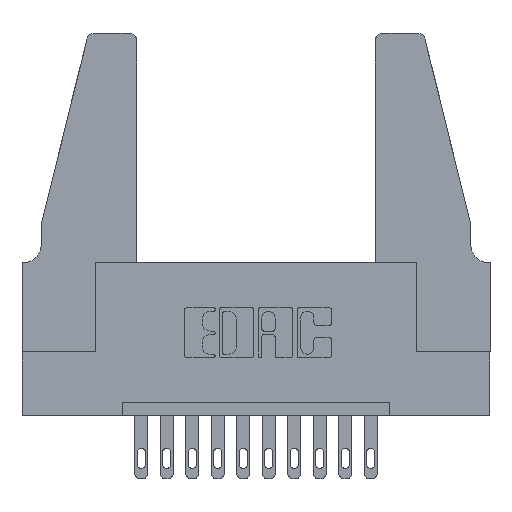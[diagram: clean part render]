
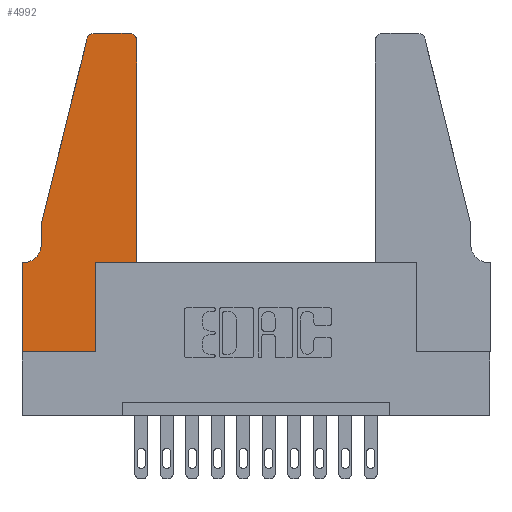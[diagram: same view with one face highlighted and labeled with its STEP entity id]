
A CAD part, top view. The second image highlights one B-rep face of the part: STEP entity #4992.
In plain terms, the highlighted planar face has unit normal (0, 0, 1).
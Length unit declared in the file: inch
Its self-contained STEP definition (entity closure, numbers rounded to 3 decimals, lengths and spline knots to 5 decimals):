
#317 = EDGE_LOOP ( 'NONE', ( #1395, #3519, #5542, #6580, #8007, #12142, #10246, #6247, #4694, #13331, #13480, #3864 ) ) ;
#408 = CARTESIAN_POINT ( 'NONE',  ( 0., 0.35, 0.37 ) ) ;
#472 = LINE ( 'NONE', #2294, #2865 ) ;
#598 = EDGE_CURVE ( 'NONE', #11204, #2477, #13326, .T. ) ;
#665 = EDGE_CURVE ( 'NONE', #9287, #4474, #9991, .T. ) ;
#851 = VECTOR ( 'NONE', #13120, 39.37008 ) ;
#853 = VECTOR ( 'NONE', #7889, 39.37008 ) ;
#1006 = DIRECTION ( 'NONE',  ( -1., 0., 0. ) ) ;
#1030 = EDGE_CURVE ( 'NONE', #8164, #5108, #3789, .T. ) ;
#1097 = CARTESIAN_POINT ( 'NONE',  ( 0.2865, 0.35, 0.37 ) ) ;
#1222 = DIRECTION ( 'NONE',  ( 0., -1., 0. ) ) ;
#1226 = CARTESIAN_POINT ( 'NONE',  ( 0.25487, 1.22718, 0.37 ) ) ;
#1299 = CARTESIAN_POINT ( 'NONE',  ( 0.2605, 1.25, 0.37 ) ) ;
#1341 = CARTESIAN_POINT ( 'NONE',  ( 0.4205, 1.25, 0.37 ) ) ;
#1350 = DIRECTION ( 'NONE',  ( -1., 0., 0. ) ) ;
#1395 = ORIENTED_EDGE ( 'NONE', *, *, #1030, .T. ) ;
#1407 = VERTEX_POINT ( 'NONE', #7362 ) ;
#1557 = CARTESIAN_POINT ( 'NONE',  ( 0., 0., 0.37 ) ) ;
#1615 = VERTEX_POINT ( 'NONE', #1226 ) ;
#1928 = VECTOR ( 'NONE', #12674, 39.37008 ) ;
#2141 = VERTEX_POINT ( 'NONE', #2352 ) ;
#2143 = CIRCLE ( 'NONE', #5082, 0.07 ) ;
#2294 = CARTESIAN_POINT ( 'NONE',  ( 0.0755, 0.5, 0.37 ) ) ;
#2352 = CARTESIAN_POINT ( 'NONE',  ( 0.0755, 0.5, 0.37 ) ) ;
#2477 = VERTEX_POINT ( 'NONE', #12676 ) ;
#2831 = DIRECTION ( 'NONE',  ( 1., 0., 0. ) ) ;
#2865 = VECTOR ( 'NONE', #1222, 39.37008 ) ;
#2970 = EDGE_CURVE ( 'NONE', #2477, #6787, #6252, .T. ) ;
#3180 = DIRECTION ( 'NONE',  ( 0., 0., 1. ) ) ;
#3229 = LINE ( 'NONE', #3492, #853 ) ;
#3268 = EDGE_CURVE ( 'NONE', #1615, #2141, #9813, .T. ) ;
#3292 = CARTESIAN_POINT ( 'NONE',  ( 0.0055, 0.42, 0.37 ) ) ;
#3492 = CARTESIAN_POINT ( 'NONE',  ( 0.4505, 0.35, 0.37 ) ) ;
#3519 = ORIENTED_EDGE ( 'NONE', *, *, #11534, .T. ) ;
#3631 = DIRECTION ( 'NONE',  ( -1., 0., 0. ) ) ;
#3654 = CARTESIAN_POINT ( 'NONE',  ( 0.4205, 1.22, 0.37 ) ) ;
#3789 = LINE ( 'NONE', #1299, #10139 ) ;
#3864 = ORIENTED_EDGE ( 'NONE', *, *, #13482, .T. ) ;
#3940 = LINE ( 'NONE', #5899, #7748 ) ;
#4137 = CARTESIAN_POINT ( 'NONE',  ( 0.0755, 0.5, 0.37 ) ) ;
#4387 = LINE ( 'NONE', #5667, #851 ) ;
#4416 = AXIS2_PLACEMENT_3D ( 'NONE', #13849, #3180, #9418 ) ;
#4474 = VERTEX_POINT ( 'NONE', #7382 ) ;
#4694 = ORIENTED_EDGE ( 'NONE', *, *, #665, .T. ) ;
#4734 = DIRECTION ( 'NONE',  ( 0., 0., 1. ) ) ;
#4768 = CARTESIAN_POINT ( 'NONE',  ( 0.0055, 0.35, 0.37 ) ) ;
#4992 = ADVANCED_FACE ( 'NONE', ( #7281 ), #13490, .T. ) ;
#5082 = AXIS2_PLACEMENT_3D ( 'NONE', #3292, #12758, #1006 ) ;
#5108 = VERTEX_POINT ( 'NONE', #10591 ) ;
#5246 = AXIS2_PLACEMENT_3D ( 'NONE', #3654, #4734, #6982 ) ;
#5493 = VECTOR ( 'NONE', #3631, 39.37008 ) ;
#5542 = ORIENTED_EDGE ( 'NONE', *, *, #3268, .T. ) ;
#5667 = CARTESIAN_POINT ( 'NONE',  ( 0., 0., 0.37 ) ) ;
#5899 = CARTESIAN_POINT ( 'NONE',  ( 0.4505, 0.35, 0.37 ) ) ;
#5912 = EDGE_CURVE ( 'NONE', #1407, #7059, #3229, .T. ) ;
#6142 = CARTESIAN_POINT ( 'NONE',  ( 0.0755, 0.35, 0.37 ) ) ;
#6247 = ORIENTED_EDGE ( 'NONE', *, *, #11183, .T. ) ;
#6252 = LINE ( 'NONE', #1557, #11778 ) ;
#6580 = ORIENTED_EDGE ( 'NONE', *, *, #6812, .T. ) ;
#6725 = CARTESIAN_POINT ( 'NONE',  ( 0.0755, 0.42, 0.37 ) ) ;
#6787 = VERTEX_POINT ( 'NONE', #7170 ) ;
#6812 = EDGE_CURVE ( 'NONE', #2141, #10793, #472, .T. ) ;
#6982 = DIRECTION ( 'NONE',  ( 1., 0., 0. ) ) ;
#7059 = VERTEX_POINT ( 'NONE', #10842 ) ;
#7170 = CARTESIAN_POINT ( 'NONE',  ( 0., 0., 0.37 ) ) ;
#7281 = FACE_OUTER_BOUND ( 'NONE', #317, .T. ) ;
#7362 = CARTESIAN_POINT ( 'NONE',  ( 0.4505, 0.35, 0.37 ) ) ;
#7382 = CARTESIAN_POINT ( 'NONE',  ( 0.2865, 0.35, 0.37 ) ) ;
#7748 = VECTOR ( 'NONE', #11469, 39.37008 ) ;
#7889 = DIRECTION ( 'NONE',  ( 0., 1., 0. ) ) ;
#7936 = DIRECTION ( 'NONE',  ( 0., 0., 1. ) ) ;
#8007 = ORIENTED_EDGE ( 'NONE', *, *, #8255, .T. ) ;
#8164 = VERTEX_POINT ( 'NONE', #1341 ) ;
#8255 = EDGE_CURVE ( 'NONE', #10793, #11204, #2143, .T. ) ;
#8609 = DIRECTION ( 'NONE',  ( 0., 1., 0. ) ) ;
#9058 = DIRECTION ( 'NONE',  ( 0., -1., 0. ) ) ;
#9180 = CIRCLE ( 'NONE', #5246, 0.03 ) ;
#9287 = VERTEX_POINT ( 'NONE', #9383 ) ;
#9383 = CARTESIAN_POINT ( 'NONE',  ( 0.2865, 0., 0.37 ) ) ;
#9418 = DIRECTION ( 'NONE',  ( 1., 0., 0. ) ) ;
#9532 = EDGE_CURVE ( 'NONE', #4474, #1407, #3940, .T. ) ;
#9813 = LINE ( 'NONE', #4137, #1928 ) ;
#9897 = AXIS2_PLACEMENT_3D ( 'NONE', #408, #7936, #2831 ) ;
#9991 = LINE ( 'NONE', #1097, #10669 ) ;
#10139 = VECTOR ( 'NONE', #1350, 39.37008 ) ;
#10246 = ORIENTED_EDGE ( 'NONE', *, *, #2970, .T. ) ;
#10591 = CARTESIAN_POINT ( 'NONE',  ( 0.284, 1.25, 0.37 ) ) ;
#10669 = VECTOR ( 'NONE', #8609, 39.37008 ) ;
#10793 = VERTEX_POINT ( 'NONE', #6725 ) ;
#10842 = CARTESIAN_POINT ( 'NONE',  ( 0.4505, 1.22, 0.37 ) ) ;
#11183 = EDGE_CURVE ( 'NONE', #6787, #9287, #4387, .T. ) ;
#11204 = VERTEX_POINT ( 'NONE', #4768 ) ;
#11469 = DIRECTION ( 'NONE',  ( 1., 0., 0. ) ) ;
#11534 = EDGE_CURVE ( 'NONE', #5108, #1615, #11580, .T. ) ;
#11580 = CIRCLE ( 'NONE', #4416, 0.03 ) ;
#11778 = VECTOR ( 'NONE', #9058, 39.37008 ) ;
#12142 = ORIENTED_EDGE ( 'NONE', *, *, #598, .T. ) ;
#12674 = DIRECTION ( 'NONE',  ( -0.239, -0.971, 0. ) ) ;
#12676 = CARTESIAN_POINT ( 'NONE',  ( 0., 0.35, 0.37 ) ) ;
#12758 = DIRECTION ( 'NONE',  ( 0., 0., -1. ) ) ;
#13120 = DIRECTION ( 'NONE',  ( 1., 0., 0. ) ) ;
#13326 = LINE ( 'NONE', #6142, #5493 ) ;
#13331 = ORIENTED_EDGE ( 'NONE', *, *, #9532, .T. ) ;
#13480 = ORIENTED_EDGE ( 'NONE', *, *, #5912, .T. ) ;
#13482 = EDGE_CURVE ( 'NONE', #7059, #8164, #9180, .T. ) ;
#13490 = PLANE ( 'NONE',  #9897 ) ;
#13849 = CARTESIAN_POINT ( 'NONE',  ( 0.284, 1.22, 0.37 ) ) ;
